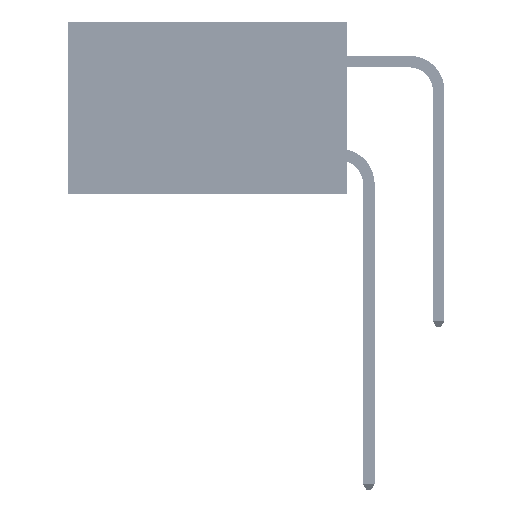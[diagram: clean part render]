
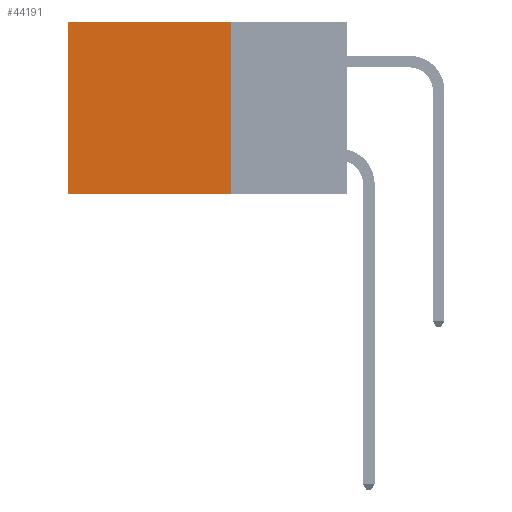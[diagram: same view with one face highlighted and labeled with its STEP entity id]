
A CAD part, left-side view. The second image highlights one B-rep face of the part: STEP entity #44191.
In plain terms, the highlighted planar face has unit normal (-1, 0, 0).
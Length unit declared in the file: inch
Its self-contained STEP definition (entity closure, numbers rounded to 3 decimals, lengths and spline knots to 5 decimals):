
#1189 = EDGE_CURVE ( 'NONE', #53118, #5287, #10325, .T. ) ;
#3569 = PLANE ( 'NONE',  #6568 ) ;
#5287 = VERTEX_POINT ( 'NONE', #49236 ) ;
#6568 = AXIS2_PLACEMENT_3D ( 'NONE', #44560, #23959, #36405 ) ;
#6780 = VECTOR ( 'NONE', #7042, 39.37008 ) ;
#7042 = DIRECTION ( 'NONE',  ( 0., 0., -1. ) ) ;
#7237 = EDGE_LOOP ( 'NONE', ( #50436, #29807, #23898, #15665 ) ) ;
#8299 = CARTESIAN_POINT ( 'NONE',  ( 0.2875, 0.6, -0.37 ) ) ;
#10325 = LINE ( 'NONE', #46491, #52996 ) ;
#13201 = EDGE_CURVE ( 'NONE', #53118, #13232, #20360, .T. ) ;
#13232 = VERTEX_POINT ( 'NONE', #31649 ) ;
#14542 = FACE_OUTER_BOUND ( 'NONE', #7237, .T. ) ;
#15166 = CARTESIAN_POINT ( 'NONE',  ( 0.2875, 0.6, 0. ) ) ;
#15665 = ORIENTED_EDGE ( 'NONE', *, *, #1189, .T. ) ;
#20360 = LINE ( 'NONE', #32015, #6780 ) ;
#22001 = DIRECTION ( 'NONE',  ( 0., 1., 0. ) ) ;
#23898 = ORIENTED_EDGE ( 'NONE', *, *, #13201, .F. ) ;
#23959 = DIRECTION ( 'NONE',  ( 1., 0., 0. ) ) ;
#25393 = DIRECTION ( 'NONE',  ( 0., 1., 0. ) ) ;
#27763 = VERTEX_POINT ( 'NONE', #8299 ) ;
#29265 = LINE ( 'NONE', #34449, #51936 ) ;
#29807 = ORIENTED_EDGE ( 'NONE', *, *, #45879, .F. ) ;
#30498 = CARTESIAN_POINT ( 'NONE',  ( 0.2875, 0.25, 0. ) ) ;
#31649 = CARTESIAN_POINT ( 'NONE',  ( 0.2875, 0.25, -0.37 ) ) ;
#32015 = CARTESIAN_POINT ( 'NONE',  ( 0.2875, 0.25, 0. ) ) ;
#34449 = CARTESIAN_POINT ( 'NONE',  ( 0.2875, 0.25, -0.37 ) ) ;
#36405 = DIRECTION ( 'NONE',  ( 0., 0., -1. ) ) ;
#41332 = LINE ( 'NONE', #15166, #49732 ) ;
#44191 = ADVANCED_FACE ( 'NONE', ( #14542 ), #3569, .F. ) ;
#44560 = CARTESIAN_POINT ( 'NONE',  ( 0.2875, 0.25, 0. ) ) ;
#45879 = EDGE_CURVE ( 'NONE', #13232, #27763, #29265, .T. ) ;
#46491 = CARTESIAN_POINT ( 'NONE',  ( 0.2875, 0.25, 0. ) ) ;
#47504 = EDGE_CURVE ( 'NONE', #5287, #27763, #41332, .T. ) ;
#49236 = CARTESIAN_POINT ( 'NONE',  ( 0.2875, 0.6, 0. ) ) ;
#49732 = VECTOR ( 'NONE', #52049, 39.37008 ) ;
#50436 = ORIENTED_EDGE ( 'NONE', *, *, #47504, .T. ) ;
#51936 = VECTOR ( 'NONE', #22001, 39.37008 ) ;
#52049 = DIRECTION ( 'NONE',  ( 0., 0., -1. ) ) ;
#52996 = VECTOR ( 'NONE', #25393, 39.37008 ) ;
#53118 = VERTEX_POINT ( 'NONE', #30498 ) ;
